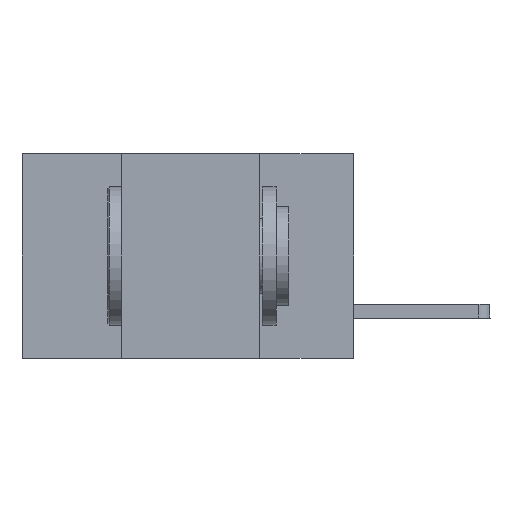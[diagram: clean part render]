
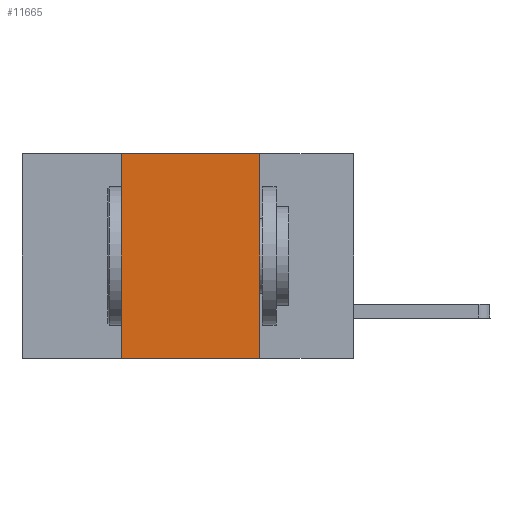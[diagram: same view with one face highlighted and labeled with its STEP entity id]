
A CAD part, left-side view. The second image highlights one B-rep face of the part: STEP entity #11665.
In plain terms, the highlighted planar face has unit normal (-1, 0, 0).
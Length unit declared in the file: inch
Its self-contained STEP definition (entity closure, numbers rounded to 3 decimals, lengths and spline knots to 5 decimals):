
#142 = DIRECTION ( 'NONE',  ( 0., 0., 1. ) ) ;
#1271 = CARTESIAN_POINT ( 'NONE',  ( 0., 0.6, 0. ) ) ;
#1324 = ORIENTED_EDGE ( 'NONE', *, *, #4654, .F. ) ;
#2263 = CARTESIAN_POINT ( 'NONE',  ( 0., 0.17, -0.37 ) ) ;
#2781 = VECTOR ( 'NONE', #142, 39.37008 ) ;
#3326 = FACE_OUTER_BOUND ( 'NONE', #13443, .T. ) ;
#3404 = DIRECTION ( 'NONE',  ( 0., 0., -1. ) ) ;
#4344 = CARTESIAN_POINT ( 'NONE',  ( 0., 0.17, 0. ) ) ;
#4353 = VECTOR ( 'NONE', #9285, 39.37008 ) ;
#4442 = CARTESIAN_POINT ( 'NONE',  ( 0., 0.42, 0. ) ) ;
#4570 = EDGE_CURVE ( 'NONE', #6897, #12860, #11467, .T. ) ;
#4654 = EDGE_CURVE ( 'NONE', #5060, #12860, #9535, .T. ) ;
#4897 = CARTESIAN_POINT ( 'NONE',  ( 0., 0.6, -0.37 ) ) ;
#5060 = VERTEX_POINT ( 'NONE', #4344 ) ;
#5177 = ORIENTED_EDGE ( 'NONE', *, *, #4570, .T. ) ;
#5217 = LINE ( 'NONE', #7076, #7818 ) ;
#5303 = EDGE_CURVE ( 'NONE', #6897, #10043, #11617, .T. ) ;
#6897 = VERTEX_POINT ( 'NONE', #14393 ) ;
#7076 = CARTESIAN_POINT ( 'NONE',  ( 0., 0.6, 0. ) ) ;
#7196 = DIRECTION ( 'NONE',  ( 0., -1., 0. ) ) ;
#7818 = VECTOR ( 'NONE', #11519, 39.37008 ) ;
#7895 = PLANE ( 'NONE',  #13052 ) ;
#8990 = DIRECTION ( 'NONE',  ( 1., 0., 0. ) ) ;
#9285 = DIRECTION ( 'NONE',  ( 0., 0., -1. ) ) ;
#9535 = LINE ( 'NONE', #12870, #4353 ) ;
#10043 = VERTEX_POINT ( 'NONE', #10104 ) ;
#10104 = CARTESIAN_POINT ( 'NONE',  ( 0., 0.42, 0. ) ) ;
#10436 = VECTOR ( 'NONE', #7196, 39.37008 ) ;
#11467 = LINE ( 'NONE', #4897, #10436 ) ;
#11519 = DIRECTION ( 'NONE',  ( 0., -1., 0. ) ) ;
#11617 = LINE ( 'NONE', #4442, #2781 ) ;
#11623 = ORIENTED_EDGE ( 'NONE', *, *, #11792, .F. ) ;
#11665 = ADVANCED_FACE ( 'NONE', ( #3326 ), #7895, .F. ) ;
#11792 = EDGE_CURVE ( 'NONE', #10043, #5060, #5217, .T. ) ;
#12860 = VERTEX_POINT ( 'NONE', #2263 ) ;
#12870 = CARTESIAN_POINT ( 'NONE',  ( 0., 0.17, 0. ) ) ;
#13052 = AXIS2_PLACEMENT_3D ( 'NONE', #1271, #8990, #3404 ) ;
#13443 = EDGE_LOOP ( 'NONE', ( #1324, #11623, #13532, #5177 ) ) ;
#13532 = ORIENTED_EDGE ( 'NONE', *, *, #5303, .F. ) ;
#14393 = CARTESIAN_POINT ( 'NONE',  ( 0., 0.42, -0.37 ) ) ;
